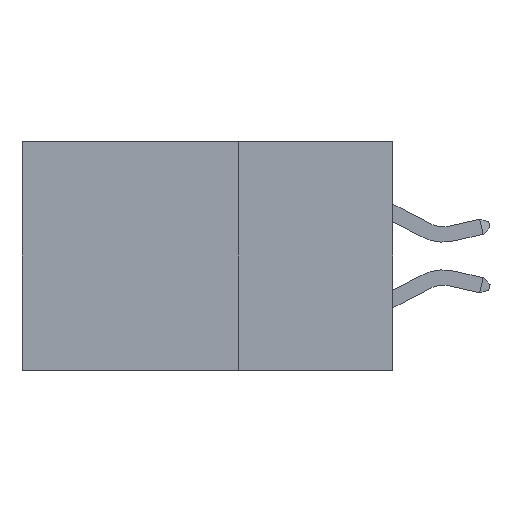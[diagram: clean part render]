
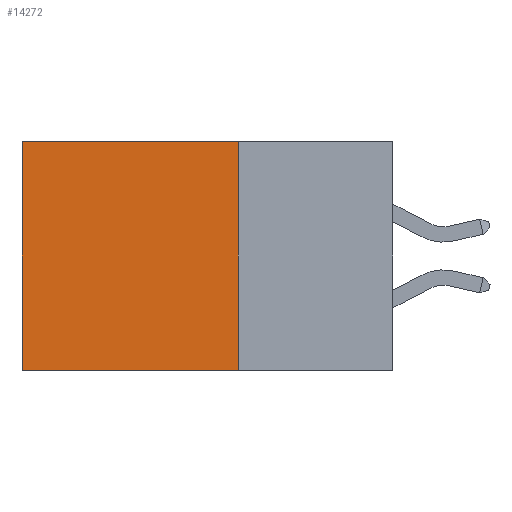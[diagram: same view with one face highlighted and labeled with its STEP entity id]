
A CAD part, left-side view. The second image highlights one B-rep face of the part: STEP entity #14272.
In plain terms, the highlighted planar face has unit normal (-1, 0, 0).
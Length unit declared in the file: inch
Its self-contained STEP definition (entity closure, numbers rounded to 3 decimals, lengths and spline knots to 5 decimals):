
#858 = ORIENTED_EDGE ( 'NONE', *, *, #5046, .F. ) ;
#1095 = VECTOR ( 'NONE', #12530, 39.37008 ) ;
#1328 = EDGE_CURVE ( 'NONE', #5246, #1989, #3002, .T. ) ;
#1429 = CARTESIAN_POINT ( 'NONE',  ( 0.2875, 0.25, 0. ) ) ;
#1989 = VERTEX_POINT ( 'NONE', #5266 ) ;
#2691 = AXIS2_PLACEMENT_3D ( 'NONE', #12868, #13974, #9639 ) ;
#2895 = LINE ( 'NONE', #14220, #11218 ) ;
#3002 = LINE ( 'NONE', #1429, #1095 ) ;
#3111 = DIRECTION ( 'NONE',  ( 0., 1., 0. ) ) ;
#3226 = VERTEX_POINT ( 'NONE', #11477 ) ;
#3336 = CARTESIAN_POINT ( 'NONE',  ( 0.2875, 0.6, 0. ) ) ;
#4043 = PLANE ( 'NONE',  #2691 ) ;
#4367 = DIRECTION ( 'NONE',  ( 0., 1., 0. ) ) ;
#5046 = EDGE_CURVE ( 'NONE', #1989, #3226, #13408, .T. ) ;
#5246 = VERTEX_POINT ( 'NONE', #13924 ) ;
#5266 = CARTESIAN_POINT ( 'NONE',  ( 0.2875, 0.25, -0.37 ) ) ;
#5727 = EDGE_CURVE ( 'NONE', #14048, #3226, #2895, .T. ) ;
#5840 = ORIENTED_EDGE ( 'NONE', *, *, #1328, .F. ) ;
#6973 = ORIENTED_EDGE ( 'NONE', *, *, #5727, .T. ) ;
#7616 = DIRECTION ( 'NONE',  ( 0., 0., -1. ) ) ;
#8666 = EDGE_LOOP ( 'NONE', ( #6973, #858, #5840, #9312 ) ) ;
#9027 = LINE ( 'NONE', #11885, #13507 ) ;
#9163 = FACE_OUTER_BOUND ( 'NONE', #8666, .T. ) ;
#9312 = ORIENTED_EDGE ( 'NONE', *, *, #9407, .T. ) ;
#9407 = EDGE_CURVE ( 'NONE', #5246, #14048, #9027, .T. ) ;
#9639 = DIRECTION ( 'NONE',  ( 0., 0., -1. ) ) ;
#11218 = VECTOR ( 'NONE', #7616, 39.37008 ) ;
#11477 = CARTESIAN_POINT ( 'NONE',  ( 0.2875, 0.6, -0.37 ) ) ;
#11885 = CARTESIAN_POINT ( 'NONE',  ( 0.2875, 0.25, 0. ) ) ;
#12530 = DIRECTION ( 'NONE',  ( 0., 0., -1. ) ) ;
#12868 = CARTESIAN_POINT ( 'NONE',  ( 0.2875, 0.25, 0. ) ) ;
#13246 = VECTOR ( 'NONE', #3111, 39.37008 ) ;
#13408 = LINE ( 'NONE', #14307, #13246 ) ;
#13507 = VECTOR ( 'NONE', #4367, 39.37008 ) ;
#13924 = CARTESIAN_POINT ( 'NONE',  ( 0.2875, 0.25, 0. ) ) ;
#13974 = DIRECTION ( 'NONE',  ( 1., 0., 0. ) ) ;
#14048 = VERTEX_POINT ( 'NONE', #3336 ) ;
#14220 = CARTESIAN_POINT ( 'NONE',  ( 0.2875, 0.6, 0. ) ) ;
#14272 = ADVANCED_FACE ( 'NONE', ( #9163 ), #4043, .F. ) ;
#14307 = CARTESIAN_POINT ( 'NONE',  ( 0.2875, 0.25, -0.37 ) ) ;
